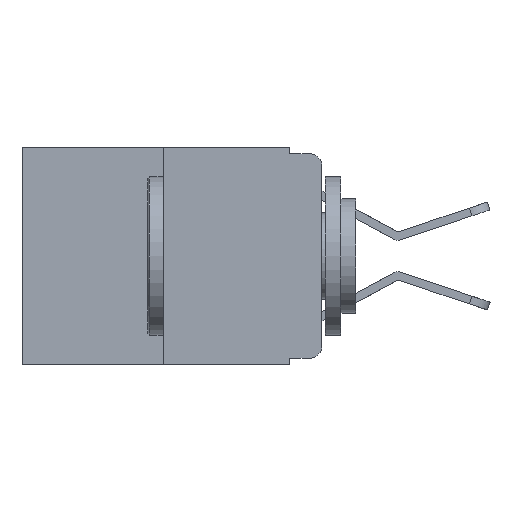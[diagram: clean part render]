
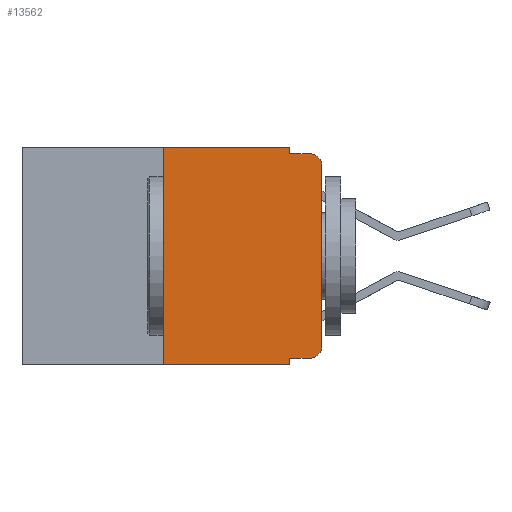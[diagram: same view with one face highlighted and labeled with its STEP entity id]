
A CAD part, left-side view. The second image highlights one B-rep face of the part: STEP entity #13562.
In plain terms, the highlighted planar face has unit normal (-1, 0, 0).
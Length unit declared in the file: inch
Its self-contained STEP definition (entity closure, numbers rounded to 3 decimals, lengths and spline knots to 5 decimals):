
#194 = EDGE_CURVE ( 'NONE', #10071, #6042, #5692, .T. ) ;
#227 = LINE ( 'NONE', #12217, #8906 ) ;
#352 = CARTESIAN_POINT ( 'NONE',  ( 0., 0.051, 0. ) ) ;
#1061 = EDGE_CURVE ( 'NONE', #10185, #1979, #8961, .T. ) ;
#1080 = CARTESIAN_POINT ( 'NONE',  ( 0., 0.051, -0.333 ) ) ;
#1327 = CIRCLE ( 'NONE', #7268, 0.02 ) ;
#1569 = PLANE ( 'NONE',  #12002 ) ;
#1708 = DIRECTION ( 'NONE',  ( -1., 0., 0. ) ) ;
#1979 = VERTEX_POINT ( 'NONE', #10015 ) ;
#2283 = VECTOR ( 'NONE', #3730, 39.37008 ) ;
#2540 = VERTEX_POINT ( 'NONE', #11237 ) ;
#2654 = CARTESIAN_POINT ( 'NONE',  ( 0., 0.02, -0.313 ) ) ;
#2675 = EDGE_CURVE ( 'NONE', #2540, #3836, #10073, .T. ) ;
#2741 = DIRECTION ( 'NONE',  ( 0., 0., 1. ) ) ;
#3157 = DIRECTION ( 'NONE',  ( -1., 0., 0. ) ) ;
#3334 = EDGE_CURVE ( 'NONE', #2540, #10071, #227, .T. ) ;
#3730 = DIRECTION ( 'NONE',  ( 0., 0., 1. ) ) ;
#3836 = VERTEX_POINT ( 'NONE', #13266 ) ;
#3885 = EDGE_LOOP ( 'NONE', ( #4208, #10240, #11704, #10688, #8888, #10030, #10560, #4633, #5865, #4019 ) ) ;
#4019 = ORIENTED_EDGE ( 'NONE', *, *, #12801, .T. ) ;
#4055 = FACE_OUTER_BOUND ( 'NONE', #3885, .T. ) ;
#4208 = ORIENTED_EDGE ( 'NONE', *, *, #4397, .T. ) ;
#4397 = EDGE_CURVE ( 'NONE', #8701, #5804, #10671, .T. ) ;
#4550 = CARTESIAN_POINT ( 'NONE',  ( 0., 0.051, 0. ) ) ;
#4633 = ORIENTED_EDGE ( 'NONE', *, *, #5449, .F. ) ;
#4764 = CARTESIAN_POINT ( 'NONE',  ( 0., 0.25, 0. ) ) ;
#4939 = VERTEX_POINT ( 'NONE', #1080 ) ;
#5242 = VECTOR ( 'NONE', #9701, 39.37008 ) ;
#5332 = VECTOR ( 'NONE', #9314, 39.37008 ) ;
#5449 = EDGE_CURVE ( 'NONE', #4939, #3836, #6252, .T. ) ;
#5477 = LINE ( 'NONE', #14916, #15189 ) ;
#5692 = LINE ( 'NONE', #7830, #15142 ) ;
#5804 = VERTEX_POINT ( 'NONE', #12773 ) ;
#5865 = ORIENTED_EDGE ( 'NONE', *, *, #14599, .T. ) ;
#6042 = VERTEX_POINT ( 'NONE', #15097 ) ;
#6252 = LINE ( 'NONE', #352, #5242 ) ;
#6693 = CARTESIAN_POINT ( 'NONE',  ( 0., 0.473, -0.343 ) ) ;
#6934 = DIRECTION ( 'NONE',  ( 0., 0., -1. ) ) ;
#7268 = AXIS2_PLACEMENT_3D ( 'NONE', #13784, #3157, #6934 ) ;
#7383 = CARTESIAN_POINT ( 'NONE',  ( 0., 0., -0.313 ) ) ;
#7630 = VECTOR ( 'NONE', #11512, 39.37008 ) ;
#7830 = CARTESIAN_POINT ( 'NONE',  ( 0., 0.473, 0. ) ) ;
#7902 = DIRECTION ( 'NONE',  ( 0., -1., 0. ) ) ;
#8294 = AXIS2_PLACEMENT_3D ( 'NONE', #2654, #1708, #11126 ) ;
#8351 = EDGE_CURVE ( 'NONE', #5804, #1979, #1327, .T. ) ;
#8701 = VERTEX_POINT ( 'NONE', #7383 ) ;
#8888 = ORIENTED_EDGE ( 'NONE', *, *, #194, .F. ) ;
#8906 = VECTOR ( 'NONE', #2741, 39.37008 ) ;
#8961 = LINE ( 'NONE', #12666, #7630 ) ;
#9314 = DIRECTION ( 'NONE',  ( 0., 0., -1. ) ) ;
#9524 = EDGE_CURVE ( 'NONE', #6042, #10185, #11640, .T. ) ;
#9626 = VECTOR ( 'NONE', #7902, 39.37008 ) ;
#9701 = DIRECTION ( 'NONE',  ( 0., 0., -1. ) ) ;
#9726 = VERTEX_POINT ( 'NONE', #10789 ) ;
#10015 = CARTESIAN_POINT ( 'NONE',  ( 0., 0.02, -0.01 ) ) ;
#10030 = ORIENTED_EDGE ( 'NONE', *, *, #3334, .F. ) ;
#10071 = VERTEX_POINT ( 'NONE', #4764 ) ;
#10073 = LINE ( 'NONE', #6693, #9626 ) ;
#10185 = VERTEX_POINT ( 'NONE', #10764 ) ;
#10240 = ORIENTED_EDGE ( 'NONE', *, *, #8351, .T. ) ;
#10560 = ORIENTED_EDGE ( 'NONE', *, *, #2675, .T. ) ;
#10671 = LINE ( 'NONE', #11750, #2283 ) ;
#10688 = ORIENTED_EDGE ( 'NONE', *, *, #9524, .F. ) ;
#10764 = CARTESIAN_POINT ( 'NONE',  ( 0., 0.051, -0.01 ) ) ;
#10789 = CARTESIAN_POINT ( 'NONE',  ( 0., 0.02, -0.333 ) ) ;
#11126 = DIRECTION ( 'NONE',  ( 0., 0., -1. ) ) ;
#11150 = DIRECTION ( 'NONE',  ( 1., 0., 0. ) ) ;
#11237 = CARTESIAN_POINT ( 'NONE',  ( 0., 0.25, -0.343 ) ) ;
#11333 = DIRECTION ( 'NONE',  ( 0., -1., 0. ) ) ;
#11512 = DIRECTION ( 'NONE',  ( 0., -1., 0. ) ) ;
#11640 = LINE ( 'NONE', #4550, #5332 ) ;
#11704 = ORIENTED_EDGE ( 'NONE', *, *, #1061, .F. ) ;
#11750 = CARTESIAN_POINT ( 'NONE',  ( 0., 0., 0. ) ) ;
#12002 = AXIS2_PLACEMENT_3D ( 'NONE', #13299, #11150, #14516 ) ;
#12217 = CARTESIAN_POINT ( 'NONE',  ( 0., 0.25, 0. ) ) ;
#12550 = DIRECTION ( 'NONE',  ( 0., -1., 0. ) ) ;
#12666 = CARTESIAN_POINT ( 'NONE',  ( 0., 0.051, -0.01 ) ) ;
#12744 = CIRCLE ( 'NONE', #8294, 0.02 ) ;
#12773 = CARTESIAN_POINT ( 'NONE',  ( 0., 0., -0.03 ) ) ;
#12801 = EDGE_CURVE ( 'NONE', #9726, #8701, #12744, .T. ) ;
#13266 = CARTESIAN_POINT ( 'NONE',  ( 0., 0.051, -0.343 ) ) ;
#13299 = CARTESIAN_POINT ( 'NONE',  ( 0., 0.473, 0. ) ) ;
#13562 = ADVANCED_FACE ( 'NONE', ( #4055 ), #1569, .F. ) ;
#13784 = CARTESIAN_POINT ( 'NONE',  ( 0., 0.02, -0.03 ) ) ;
#14516 = DIRECTION ( 'NONE',  ( 0., 0., -1. ) ) ;
#14599 = EDGE_CURVE ( 'NONE', #4939, #9726, #5477, .T. ) ;
#14916 = CARTESIAN_POINT ( 'NONE',  ( 0., 0.051, -0.333 ) ) ;
#15097 = CARTESIAN_POINT ( 'NONE',  ( 0., 0.051, 0. ) ) ;
#15142 = VECTOR ( 'NONE', #12550, 39.37008 ) ;
#15189 = VECTOR ( 'NONE', #11333, 39.37008 ) ;
